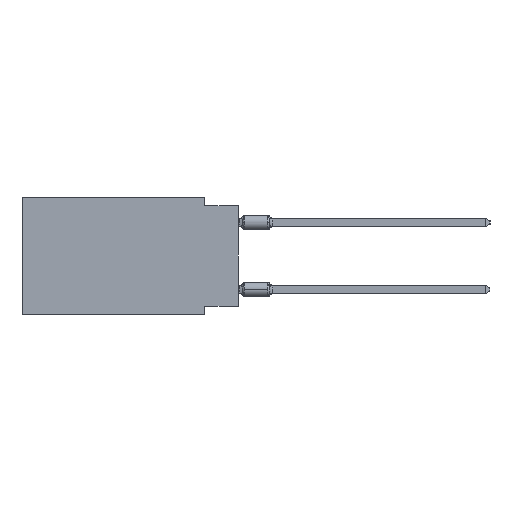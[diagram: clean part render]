
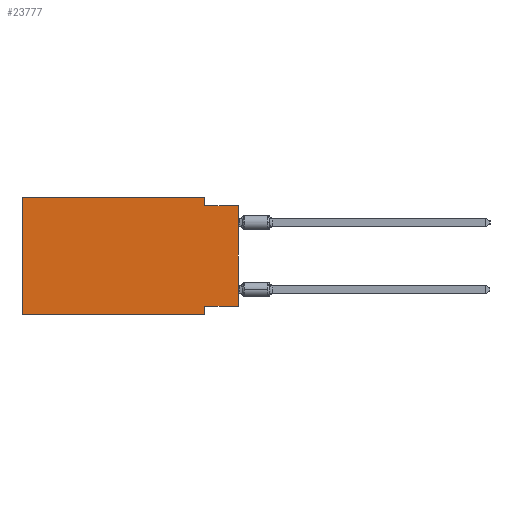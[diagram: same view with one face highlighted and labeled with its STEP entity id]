
A CAD part, left-side view. The second image highlights one B-rep face of the part: STEP entity #23777.
In plain terms, the highlighted planar face has unit normal (-1, 0, 0).
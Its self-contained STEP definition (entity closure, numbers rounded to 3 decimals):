
#2 = ORIENTED_EDGE ( 'NONE', *, *, #31052, .F. ) ;
#359 = AXIS2_PLACEMENT_3D ( 'NONE', #962, #6403, #21862 ) ;
#434 = VERTEX_POINT ( 'NONE', #17516 ) ;
#862 = LINE ( 'NONE', #3566, #27227 ) ;
#962 = CARTESIAN_POINT ( 'NONE',  ( 0., 16.383, 0. ) ) ;
#2145 = EDGE_CURVE ( 'NONE', #19256, #6380, #33427, .T. ) ;
#2941 = ORIENTED_EDGE ( 'NONE', *, *, #8602, .F. ) ;
#3151 = EDGE_CURVE ( 'NONE', #28934, #28454, #19331, .T. ) ;
#3566 = CARTESIAN_POINT ( 'NONE',  ( 0., 2.54, -8.89 ) ) ;
#3569 = VECTOR ( 'NONE', #32838, 1000. ) ;
#3884 = CARTESIAN_POINT ( 'NONE',  ( 0., 16.383, 0. ) ) ;
#4205 = CARTESIAN_POINT ( 'NONE',  ( 0., 0., -0.635 ) ) ;
#4358 = ORIENTED_EDGE ( 'NONE', *, *, #3151, .F. ) ;
#4899 = CARTESIAN_POINT ( 'NONE',  ( 0., 16.383, 0. ) ) ;
#5230 = EDGE_CURVE ( 'NONE', #15432, #15721, #33168, .T. ) ;
#6380 = VERTEX_POINT ( 'NONE', #23631 ) ;
#6403 = DIRECTION ( 'NONE',  ( 1., 0., 0. ) ) ;
#8227 = DIRECTION ( 'NONE',  ( 0., 0., -1. ) ) ;
#8572 = CARTESIAN_POINT ( 'NONE',  ( 0., 16.383, 0. ) ) ;
#8602 = EDGE_CURVE ( 'NONE', #434, #29786, #32370, .T. ) ;
#8901 = ORIENTED_EDGE ( 'NONE', *, *, #25199, .F. ) ;
#8940 = PLANE ( 'NONE',  #359 ) ;
#9392 = CARTESIAN_POINT ( 'NONE',  ( 0., 16.383, -8.89 ) ) ;
#9879 = CARTESIAN_POINT ( 'NONE',  ( 0., 16.383, -8.89 ) ) ;
#10159 = ORIENTED_EDGE ( 'NONE', *, *, #18968, .T. ) ;
#10780 = CARTESIAN_POINT ( 'NONE',  ( 0., 2.54, 0. ) ) ;
#11374 = EDGE_CURVE ( 'NONE', #29786, #15721, #862, .T. ) ;
#12333 = CARTESIAN_POINT ( 'NONE',  ( 0., 0., 0. ) ) ;
#12947 = CARTESIAN_POINT ( 'NONE',  ( 0., 2.54, -8.255 ) ) ;
#13505 = VECTOR ( 'NONE', #29306, 1000. ) ;
#14502 = ORIENTED_EDGE ( 'NONE', *, *, #5230, .T. ) ;
#15432 = VERTEX_POINT ( 'NONE', #9879 ) ;
#15721 = VERTEX_POINT ( 'NONE', #24467 ) ;
#17157 = LINE ( 'NONE', #3884, #22161 ) ;
#17428 = DIRECTION ( 'NONE',  ( 0., 0., 1. ) ) ;
#17516 = CARTESIAN_POINT ( 'NONE',  ( 0., 0., -8.255 ) ) ;
#18968 = EDGE_CURVE ( 'NONE', #434, #28454, #23017, .T. ) ;
#19094 = VECTOR ( 'NONE', #17428, 1000. ) ;
#19256 = VERTEX_POINT ( 'NONE', #8572 ) ;
#19331 = LINE ( 'NONE', #4205, #20307 ) ;
#20307 = VECTOR ( 'NONE', #32567, 1000. ) ;
#20505 = ORIENTED_EDGE ( 'NONE', *, *, #2145, .F. ) ;
#20829 = EDGE_LOOP ( 'NONE', ( #10159, #4358, #2, #20505, #8901, #14502, #29183, #2941 ) ) ;
#21862 = DIRECTION ( 'NONE',  ( 0., 0., -1. ) ) ;
#22161 = VECTOR ( 'NONE', #22404, 1000. ) ;
#22404 = DIRECTION ( 'NONE',  ( 0., 0., 1. ) ) ;
#23017 = LINE ( 'NONE', #12333, #19094 ) ;
#23348 = LINE ( 'NONE', #10780, #31202 ) ;
#23395 = DIRECTION ( 'NONE',  ( 0., -1., 0. ) ) ;
#23631 = CARTESIAN_POINT ( 'NONE',  ( 0., 2.54, 0. ) ) ;
#23777 = ADVANCED_FACE ( 'NONE', ( #32043 ), #8940, .F. ) ;
#24467 = CARTESIAN_POINT ( 'NONE',  ( 0., 2.54, -8.89 ) ) ;
#25199 = EDGE_CURVE ( 'NONE', #15432, #19256, #17157, .T. ) ;
#26769 = CARTESIAN_POINT ( 'NONE',  ( 0., 0., -8.255 ) ) ;
#27227 = VECTOR ( 'NONE', #32118, 1000. ) ;
#27867 = VECTOR ( 'NONE', #23395, 1000. ) ;
#28128 = CARTESIAN_POINT ( 'NONE',  ( 0., 2.54, -0.635 ) ) ;
#28454 = VERTEX_POINT ( 'NONE', #30374 ) ;
#28934 = VERTEX_POINT ( 'NONE', #28128 ) ;
#29183 = ORIENTED_EDGE ( 'NONE', *, *, #11374, .F. ) ;
#29306 = DIRECTION ( 'NONE',  ( 0., 1., 0. ) ) ;
#29786 = VERTEX_POINT ( 'NONE', #12947 ) ;
#30374 = CARTESIAN_POINT ( 'NONE',  ( 0., 0., -0.635 ) ) ;
#31052 = EDGE_CURVE ( 'NONE', #6380, #28934, #23348, .T. ) ;
#31202 = VECTOR ( 'NONE', #8227, 1000. ) ;
#32043 = FACE_OUTER_BOUND ( 'NONE', #20829, .T. ) ;
#32118 = DIRECTION ( 'NONE',  ( 0., 0., -1. ) ) ;
#32370 = LINE ( 'NONE', #26769, #13505 ) ;
#32567 = DIRECTION ( 'NONE',  ( 0., -1., 0. ) ) ;
#32838 = DIRECTION ( 'NONE',  ( 0., -1., 0. ) ) ;
#33168 = LINE ( 'NONE', #9392, #3569 ) ;
#33427 = LINE ( 'NONE', #4899, #27867 ) ;
